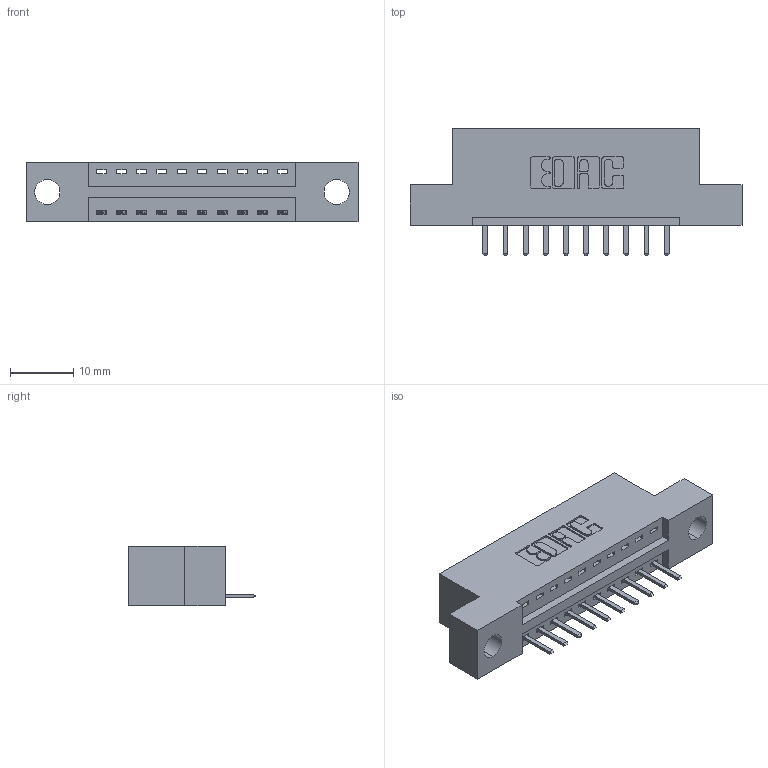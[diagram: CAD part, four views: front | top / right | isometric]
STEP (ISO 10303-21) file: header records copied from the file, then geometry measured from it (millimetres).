
FILE_DESCRIPTION (( 'STEP AP203' ), '1' );
FILE_NAME ('346-010-520-104.STEP', '2022-05-04T23:18:15', ( '' ), ( '' ), 'SwSTEP 2.0', 'SolidWorks 2020', '' );
FILE_SCHEMA (( 'CONFIG_CONTROL_DESIGN' ));
Length unit declared in the file: inch
Products named in the file (3): 346-010-520-104; 346 Part_Flush Mounting Lugs - 0.156 Dia-TH; 345-292-001_345-293-120
Assembly tree (11 placements, depth 2):
  346-010-520-104
    346 Part_Flush Mounting Lugs - 0.156 Dia-TH
    345-292-001_345-293-120  x10
Bounding box: 52.32 x 20.02 x 9.4 mm (x, y, z)
Volume: 4653.4 mm3; surface area: 5212 mm2
Topology: 11 solids, 11 shells, 756 faces, 2205 edges, 1442 vertices
Faces by surface type: plane 510, cylinder 246
Entity records: 11047 total; most frequent: CARTESIAN_POINT 1924, ORIENTED_EDGE 1854, DIRECTION 1723, EDGE_CURVE 927, LINE 751, VECTOR 751, VERTEX_POINT 614, AXIS2_PLACEMENT_3D 486
